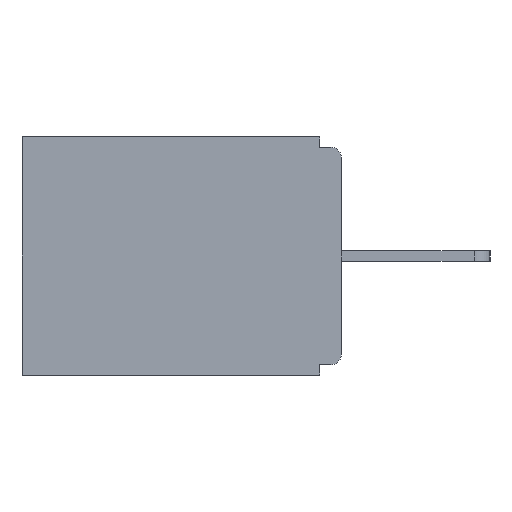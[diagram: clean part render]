
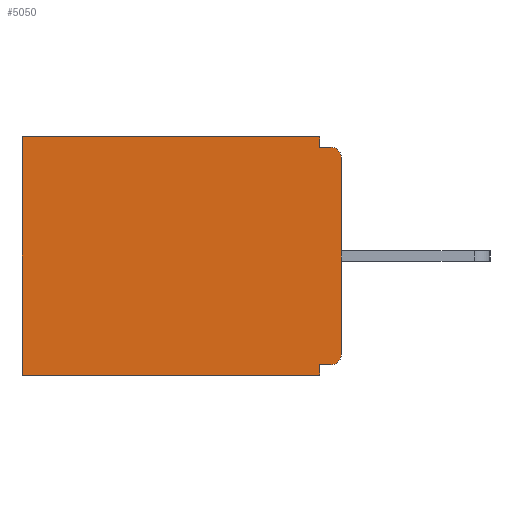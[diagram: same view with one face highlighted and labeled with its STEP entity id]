
A CAD part, left-side view. The second image highlights one B-rep face of the part: STEP entity #5050.
In plain terms, the highlighted planar face has unit normal (-1, 0, 0).
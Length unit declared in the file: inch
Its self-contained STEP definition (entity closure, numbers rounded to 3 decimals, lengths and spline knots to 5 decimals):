
#237 = CIRCLE ( 'NONE', #6680, 0.015 ) ;
#333 = LINE ( 'NONE', #13534, #3225 ) ;
#364 = DIRECTION ( 'NONE',  ( 0., 0., -1. ) ) ;
#739 = ORIENTED_EDGE ( 'NONE', *, *, #9553, .T. ) ;
#1331 = DIRECTION ( 'NONE',  ( 0., 0., -1. ) ) ;
#1359 = VERTEX_POINT ( 'NONE', #12172 ) ;
#1572 = DIRECTION ( 'NONE',  ( 0., 0., -1. ) ) ;
#1666 = VECTOR ( 'NONE', #364, 39.37008 ) ;
#1774 = VERTEX_POINT ( 'NONE', #15042 ) ;
#1810 = VERTEX_POINT ( 'NONE', #8770 ) ;
#1849 = VERTEX_POINT ( 'NONE', #5887 ) ;
#1874 = ORIENTED_EDGE ( 'NONE', *, *, #15620, .T. ) ;
#2082 = VERTEX_POINT ( 'NONE', #8844 ) ;
#2316 = ORIENTED_EDGE ( 'NONE', *, *, #14531, .F. ) ;
#3110 = CARTESIAN_POINT ( 'NONE',  ( 0.298, 0.015, -0.03 ) ) ;
#3225 = VECTOR ( 'NONE', #6274, 39.37008 ) ;
#3659 = CARTESIAN_POINT ( 'NONE',  ( 0.298, 0., 0. ) ) ;
#3837 = ORIENTED_EDGE ( 'NONE', *, *, #15955, .F. ) ;
#3993 = FACE_OUTER_BOUND ( 'NONE', #9272, .T. ) ;
#4253 = CARTESIAN_POINT ( 'NONE',  ( 0.298, 0.031, -0.343 ) ) ;
#4381 = VERTEX_POINT ( 'NONE', #13541 ) ;
#4607 = CARTESIAN_POINT ( 'NONE',  ( 0.298, 0., -0.343 ) ) ;
#4664 = LINE ( 'NONE', #9908, #11436 ) ;
#4811 = LINE ( 'NONE', #13988, #7987 ) ;
#4894 = ORIENTED_EDGE ( 'NONE', *, *, #13384, .T. ) ;
#4944 = VERTEX_POINT ( 'NONE', #4253 ) ;
#4975 = DIRECTION ( 'NONE',  ( -1., 0., 0. ) ) ;
#5050 = ADVANCED_FACE ( 'NONE', ( #3993 ), #14025, .F. ) ;
#5053 = EDGE_CURVE ( 'NONE', #1849, #1810, #237, .T. ) ;
#5335 = LINE ( 'NONE', #7240, #1666 ) ;
#5403 = LINE ( 'NONE', #8391, #12141 ) ;
#5628 = EDGE_CURVE ( 'NONE', #2082, #1810, #333, .T. ) ;
#5887 = CARTESIAN_POINT ( 'NONE',  ( 0.298, 0., -0.03 ) ) ;
#6274 = DIRECTION ( 'NONE',  ( 0., -1., 0. ) ) ;
#6512 = LINE ( 'NONE', #4607, #6906 ) ;
#6680 = AXIS2_PLACEMENT_3D ( 'NONE', #3110, #4975, #14667 ) ;
#6906 = VECTOR ( 'NONE', #16380, 39.37008 ) ;
#6944 = DIRECTION ( 'NONE',  ( -1., 0., 0. ) ) ;
#7191 = ORIENTED_EDGE ( 'NONE', *, *, #5628, .F. ) ;
#7240 = CARTESIAN_POINT ( 'NONE',  ( 0.298, 0.46, 0. ) ) ;
#7566 = AXIS2_PLACEMENT_3D ( 'NONE', #3659, #14462, #16385 ) ;
#7658 = ORIENTED_EDGE ( 'NONE', *, *, #11628, .F. ) ;
#7863 = ORIENTED_EDGE ( 'NONE', *, *, #9903, .F. ) ;
#7987 = VECTOR ( 'NONE', #14506, 39.37008 ) ;
#8067 = ORIENTED_EDGE ( 'NONE', *, *, #13205, .F. ) ;
#8301 = VECTOR ( 'NONE', #1331, 39.37008 ) ;
#8391 = CARTESIAN_POINT ( 'NONE',  ( 0.298, 0., 0. ) ) ;
#8725 = LINE ( 'NONE', #12278, #8301 ) ;
#8770 = CARTESIAN_POINT ( 'NONE',  ( 0.298, 0.015, -0.015 ) ) ;
#8844 = CARTESIAN_POINT ( 'NONE',  ( 0.298, 0.031, -0.015 ) ) ;
#9272 = EDGE_LOOP ( 'NONE', ( #10455, #7191, #8067, #739, #4894, #7863, #3837, #2316, #1874, #7658 ) ) ;
#9553 = EDGE_CURVE ( 'NONE', #14902, #13948, #4811, .T. ) ;
#9903 = EDGE_CURVE ( 'NONE', #4944, #12136, #6512, .T. ) ;
#9908 = CARTESIAN_POINT ( 'NONE',  ( 0.298, 0., -0.328 ) ) ;
#10455 = ORIENTED_EDGE ( 'NONE', *, *, #5053, .T. ) ;
#10814 = CARTESIAN_POINT ( 'NONE',  ( 0.298, 0.031, 0. ) ) ;
#10819 = AXIS2_PLACEMENT_3D ( 'NONE', #14851, #6944, #16050 ) ;
#11436 = VECTOR ( 'NONE', #12582, 39.37008 ) ;
#11628 = EDGE_CURVE ( 'NONE', #1849, #1774, #5403, .T. ) ;
#11975 = VECTOR ( 'NONE', #16664, 39.37008 ) ;
#12136 = VERTEX_POINT ( 'NONE', #14652 ) ;
#12141 = VECTOR ( 'NONE', #1572, 39.37008 ) ;
#12172 = CARTESIAN_POINT ( 'NONE',  ( 0.298, 0.015, -0.328 ) ) ;
#12278 = CARTESIAN_POINT ( 'NONE',  ( 0.298, 0.031, -0.343 ) ) ;
#12582 = DIRECTION ( 'NONE',  ( 0., 1., 0. ) ) ;
#12792 = CARTESIAN_POINT ( 'NONE',  ( 0.298, 0.46, 0. ) ) ;
#13205 = EDGE_CURVE ( 'NONE', #14902, #2082, #8725, .T. ) ;
#13384 = EDGE_CURVE ( 'NONE', #13948, #12136, #5335, .T. ) ;
#13534 = CARTESIAN_POINT ( 'NONE',  ( 0.298, 0., -0.015 ) ) ;
#13541 = CARTESIAN_POINT ( 'NONE',  ( 0.298, 0.031, -0.328 ) ) ;
#13948 = VERTEX_POINT ( 'NONE', #12792 ) ;
#13988 = CARTESIAN_POINT ( 'NONE',  ( 0.298, 0., 0. ) ) ;
#14025 = PLANE ( 'NONE',  #7566 ) ;
#14462 = DIRECTION ( 'NONE',  ( 1., 0., 0. ) ) ;
#14506 = DIRECTION ( 'NONE',  ( 0., 1., 0. ) ) ;
#14531 = EDGE_CURVE ( 'NONE', #1359, #4381, #4664, .T. ) ;
#14608 = CIRCLE ( 'NONE', #10819, 0.015 ) ;
#14652 = CARTESIAN_POINT ( 'NONE',  ( 0.298, 0.46, -0.343 ) ) ;
#14667 = DIRECTION ( 'NONE',  ( 0., 0., -1. ) ) ;
#14851 = CARTESIAN_POINT ( 'NONE',  ( 0.298, 0.015, -0.313 ) ) ;
#14902 = VERTEX_POINT ( 'NONE', #10814 ) ;
#15042 = CARTESIAN_POINT ( 'NONE',  ( 0.298, 0., -0.313 ) ) ;
#15462 = CARTESIAN_POINT ( 'NONE',  ( 0.298, 0.031, -0.343 ) ) ;
#15620 = EDGE_CURVE ( 'NONE', #1359, #1774, #14608, .T. ) ;
#15705 = LINE ( 'NONE', #15462, #11975 ) ;
#15955 = EDGE_CURVE ( 'NONE', #4381, #4944, #15705, .T. ) ;
#16050 = DIRECTION ( 'NONE',  ( 0., 0., -1. ) ) ;
#16380 = DIRECTION ( 'NONE',  ( 0., 1., 0. ) ) ;
#16385 = DIRECTION ( 'NONE',  ( 0., 0., -1. ) ) ;
#16664 = DIRECTION ( 'NONE',  ( 0., 0., -1. ) ) ;
